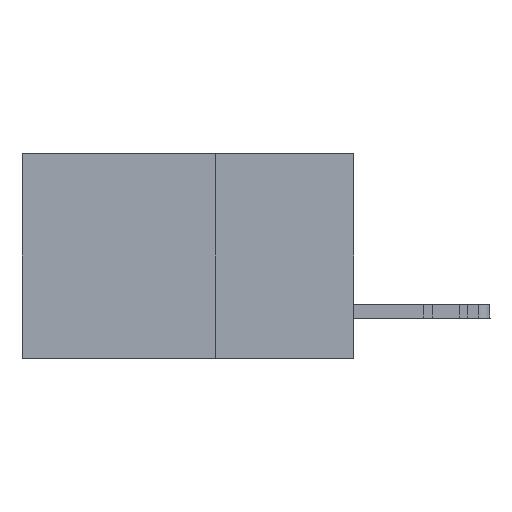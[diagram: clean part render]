
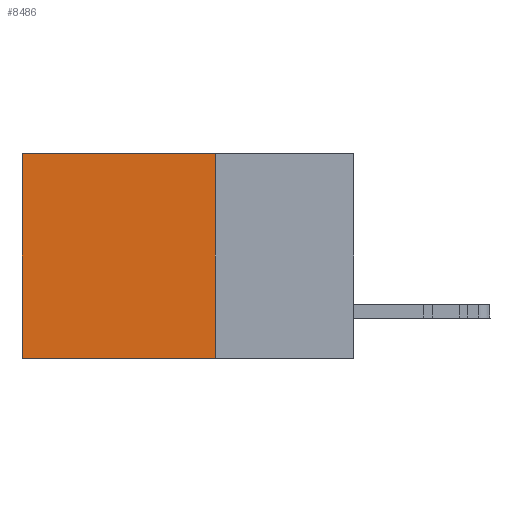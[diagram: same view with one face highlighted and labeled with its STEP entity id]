
A CAD part, left-side view. The second image highlights one B-rep face of the part: STEP entity #8486.
In plain terms, the highlighted planar face has unit normal (-1, 0, 0).
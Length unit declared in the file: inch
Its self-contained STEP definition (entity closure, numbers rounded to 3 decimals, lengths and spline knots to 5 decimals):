
#1299 = DIRECTION ( 'NONE',  ( 0., 0., -1. ) ) ;
#2315 = CARTESIAN_POINT ( 'NONE',  ( 0.2875, 0.6, 0. ) ) ;
#4437 = VECTOR ( 'NONE', #27521, 39.37008 ) ;
#7190 = LINE ( 'NONE', #7689, #27314 ) ;
#7556 = VERTEX_POINT ( 'NONE', #31482 ) ;
#7689 = CARTESIAN_POINT ( 'NONE',  ( 0.2875, 0.25, 0. ) ) ;
#8486 = ADVANCED_FACE ( 'NONE', ( #29940 ), #11610, .F. ) ;
#8838 = ORIENTED_EDGE ( 'NONE', *, *, #18528, .T. ) ;
#8858 = DIRECTION ( 'NONE',  ( 0., 0., -1. ) ) ;
#9964 = CARTESIAN_POINT ( 'NONE',  ( 0.2875, 0.25, 0. ) ) ;
#11003 = DIRECTION ( 'NONE',  ( 0., 1., 0. ) ) ;
#11610 = PLANE ( 'NONE',  #31845 ) ;
#12902 = LINE ( 'NONE', #2315, #20616 ) ;
#13619 = CARTESIAN_POINT ( 'NONE',  ( 0.2875, 0.25, -0.37 ) ) ;
#14429 = DIRECTION ( 'NONE',  ( 0., 1., 0. ) ) ;
#15566 = VERTEX_POINT ( 'NONE', #13619 ) ;
#15575 = ORIENTED_EDGE ( 'NONE', *, *, #42099, .F. ) ;
#15927 = VERTEX_POINT ( 'NONE', #42088 ) ;
#16777 = ORIENTED_EDGE ( 'NONE', *, *, #37333, .F. ) ;
#17286 = LINE ( 'NONE', #31135, #4437 ) ;
#18123 = CARTESIAN_POINT ( 'NONE',  ( 0.2875, 0.25, 0. ) ) ;
#18528 = EDGE_CURVE ( 'NONE', #32169, #7556, #7190, .T. ) ;
#20616 = VECTOR ( 'NONE', #8858, 39.37008 ) ;
#21423 = EDGE_LOOP ( 'NONE', ( #21885, #15575, #16777, #8838 ) ) ;
#21885 = ORIENTED_EDGE ( 'NONE', *, *, #27699, .T. ) ;
#24586 = DIRECTION ( 'NONE',  ( 1., 0., 0. ) ) ;
#27214 = VECTOR ( 'NONE', #14429, 39.37008 ) ;
#27314 = VECTOR ( 'NONE', #11003, 39.37008 ) ;
#27521 = DIRECTION ( 'NONE',  ( 0., 0., -1. ) ) ;
#27699 = EDGE_CURVE ( 'NONE', #7556, #15927, #12902, .T. ) ;
#29940 = FACE_OUTER_BOUND ( 'NONE', #21423, .T. ) ;
#31135 = CARTESIAN_POINT ( 'NONE',  ( 0.2875, 0.25, 0. ) ) ;
#31482 = CARTESIAN_POINT ( 'NONE',  ( 0.2875, 0.6, 0. ) ) ;
#31845 = AXIS2_PLACEMENT_3D ( 'NONE', #18123, #24586, #1299 ) ;
#32169 = VERTEX_POINT ( 'NONE', #9964 ) ;
#34158 = CARTESIAN_POINT ( 'NONE',  ( 0.2875, 0.25, -0.37 ) ) ;
#37333 = EDGE_CURVE ( 'NONE', #32169, #15566, #17286, .T. ) ;
#40045 = LINE ( 'NONE', #34158, #27214 ) ;
#42088 = CARTESIAN_POINT ( 'NONE',  ( 0.2875, 0.6, -0.37 ) ) ;
#42099 = EDGE_CURVE ( 'NONE', #15566, #15927, #40045, .T. ) ;
